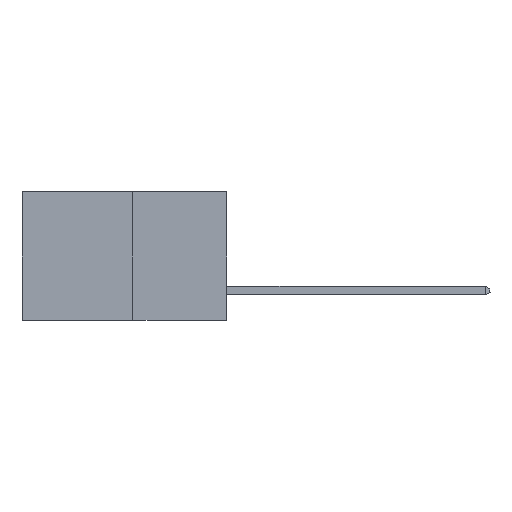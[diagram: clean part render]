
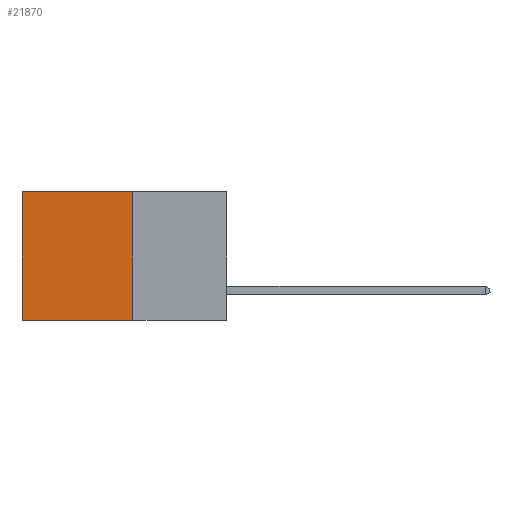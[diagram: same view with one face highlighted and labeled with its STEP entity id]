
A CAD part, left-side view. The second image highlights one B-rep face of the part: STEP entity #21870.
In plain terms, the highlighted planar face has unit normal (-1, 0, 0).
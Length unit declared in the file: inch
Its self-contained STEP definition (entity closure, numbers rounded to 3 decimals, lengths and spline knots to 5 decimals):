
#1558 = CARTESIAN_POINT ( 'NONE',  ( 0.277, 0.27, -0.37 ) ) ;
#4735 = ORIENTED_EDGE ( 'NONE', *, *, #18551, .F. ) ;
#4906 = DIRECTION ( 'NONE',  ( 0., 0., -1. ) ) ;
#5431 = LINE ( 'NONE', #31658, #19108 ) ;
#5709 = VECTOR ( 'NONE', #31856, 39.37008 ) ;
#5731 = VERTEX_POINT ( 'NONE', #6643 ) ;
#6643 = CARTESIAN_POINT ( 'NONE',  ( 0.277, 0.59, -0.37 ) ) ;
#6793 = CARTESIAN_POINT ( 'NONE',  ( 0.277, 0.27, -0.37 ) ) ;
#7027 = EDGE_CURVE ( 'NONE', #7221, #5731, #24413, .T. ) ;
#7221 = VERTEX_POINT ( 'NONE', #6793 ) ;
#8099 = VERTEX_POINT ( 'NONE', #10910 ) ;
#10776 = EDGE_LOOP ( 'NONE', ( #15827, #22671, #4735, #13352 ) ) ;
#10910 = CARTESIAN_POINT ( 'NONE',  ( 0.277, 0.27, 0. ) ) ;
#11425 = DIRECTION ( 'NONE',  ( 0., 1., 0. ) ) ;
#11864 = DIRECTION ( 'NONE',  ( 0., 1., 0. ) ) ;
#12188 = VERTEX_POINT ( 'NONE', #29661 ) ;
#13352 = ORIENTED_EDGE ( 'NONE', *, *, #22961, .T. ) ;
#15827 = ORIENTED_EDGE ( 'NONE', *, *, #16143, .T. ) ;
#16143 = EDGE_CURVE ( 'NONE', #12188, #5731, #5431, .T. ) ;
#17801 = CARTESIAN_POINT ( 'NONE',  ( 0.277, 0.27, -0.37 ) ) ;
#18551 = EDGE_CURVE ( 'NONE', #8099, #7221, #25877, .T. ) ;
#18697 = VECTOR ( 'NONE', #11425, 39.37008 ) ;
#19108 = VECTOR ( 'NONE', #29144, 39.37008 ) ;
#20252 = DIRECTION ( 'NONE',  ( 1., 0., 0. ) ) ;
#21806 = CARTESIAN_POINT ( 'NONE',  ( 0.277, 0.27, 0. ) ) ;
#21870 = ADVANCED_FACE ( 'NONE', ( #32657 ), #32543, .F. ) ;
#22671 = ORIENTED_EDGE ( 'NONE', *, *, #7027, .F. ) ;
#22961 = EDGE_CURVE ( 'NONE', #8099, #12188, #29839, .T. ) ;
#23307 = VECTOR ( 'NONE', #11864, 39.37008 ) ;
#24413 = LINE ( 'NONE', #26298, #18697 ) ;
#24475 = AXIS2_PLACEMENT_3D ( 'NONE', #17801, #20252, #4906 ) ;
#25877 = LINE ( 'NONE', #1558, #5709 ) ;
#26298 = CARTESIAN_POINT ( 'NONE',  ( 0.277, 0.27, -0.37 ) ) ;
#29144 = DIRECTION ( 'NONE',  ( 0., 0., -1. ) ) ;
#29661 = CARTESIAN_POINT ( 'NONE',  ( 0.277, 0.59, 0. ) ) ;
#29839 = LINE ( 'NONE', #21806, #23307 ) ;
#31658 = CARTESIAN_POINT ( 'NONE',  ( 0.277, 0.59, -0.37 ) ) ;
#31856 = DIRECTION ( 'NONE',  ( 0., 0., -1. ) ) ;
#32543 = PLANE ( 'NONE',  #24475 ) ;
#32657 = FACE_OUTER_BOUND ( 'NONE', #10776, .T. ) ;
